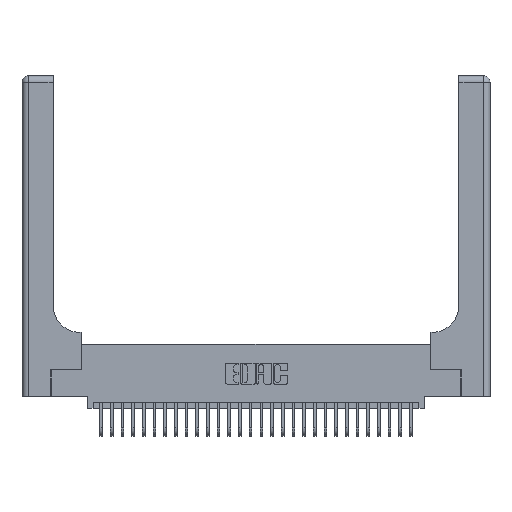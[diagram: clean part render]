
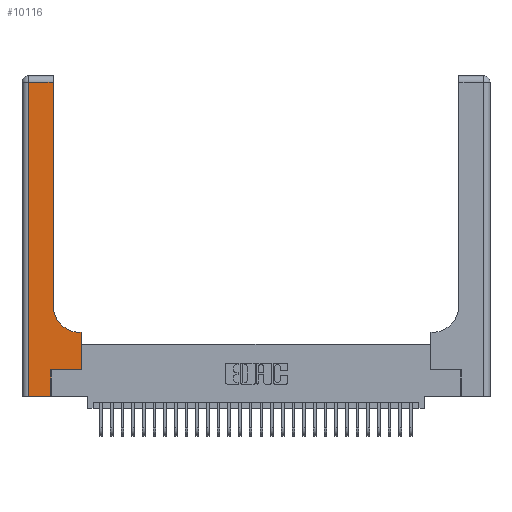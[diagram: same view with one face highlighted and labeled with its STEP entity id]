
A CAD part, top view. The second image highlights one B-rep face of the part: STEP entity #10116.
In plain terms, the highlighted planar face has unit normal (0, 0, 1).
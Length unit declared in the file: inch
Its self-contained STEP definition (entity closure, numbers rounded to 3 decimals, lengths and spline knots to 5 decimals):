
#87 = EDGE_CURVE ( 'NONE', #29212, #15285, #19806, .T. ) ;
#368 = VERTEX_POINT ( 'NONE', #7035 ) ;
#499 = EDGE_CURVE ( 'NONE', #4516, #5817, #8561, .T. ) ;
#904 = ORIENTED_EDGE ( 'NONE', *, *, #6698, .T. ) ;
#1080 = ORIENTED_EDGE ( 'NONE', *, *, #13180, .T. ) ;
#1285 = CARTESIAN_POINT ( 'NONE',  ( 0.5585, 0.6, 0.37 ) ) ;
#1563 = CARTESIAN_POINT ( 'NONE',  ( 0.5415, 0.6, 0.37 ) ) ;
#2894 = DIRECTION ( 'NONE',  ( 0., 0., -1. ) ) ;
#2907 = VERTEX_POINT ( 'NONE', #31944 ) ;
#3461 = DIRECTION ( 'NONE',  ( -1., 0., 0. ) ) ;
#3591 = CARTESIAN_POINT ( 'NONE',  ( 0.5415, 0.85, 0.37 ) ) ;
#4261 = EDGE_CURVE ( 'NONE', #13746, #29212, #31647, .T. ) ;
#4516 = VERTEX_POINT ( 'NONE', #1285 ) ;
#4831 = CARTESIAN_POINT ( 'NONE',  ( 0., 2.94, 0.37 ) ) ;
#5466 = DIRECTION ( 'NONE',  ( 0., -1., 0. ) ) ;
#5582 = VECTOR ( 'NONE', #17116, 39.37008 ) ;
#5611 = CARTESIAN_POINT ( 'NONE',  ( 0., 3., 0.37 ) ) ;
#5817 = VERTEX_POINT ( 'NONE', #1563 ) ;
#6345 = ORIENTED_EDGE ( 'NONE', *, *, #29522, .T. ) ;
#6505 = AXIS2_PLACEMENT_3D ( 'NONE', #5611, #2894, #20474 ) ;
#6698 = EDGE_CURVE ( 'NONE', #368, #2907, #15190, .T. ) ;
#6971 = CARTESIAN_POINT ( 'NONE',  ( 0.2915, 3., 0.37 ) ) ;
#7035 = CARTESIAN_POINT ( 'NONE',  ( 0.269, 0., 0.37 ) ) ;
#7038 = VERTEX_POINT ( 'NONE', #13285 ) ;
#7787 = VECTOR ( 'NONE', #3461, 39.37008 ) ;
#7920 = EDGE_LOOP ( 'NONE', ( #15923, #23489, #28900, #8496, #904, #1080, #6345, #16063, #27924 ) ) ;
#8440 = CARTESIAN_POINT ( 'NONE',  ( 0.06, 0., 0.37 ) ) ;
#8454 = DIRECTION ( 'NONE',  ( 1., 0., 0. ) ) ;
#8496 = ORIENTED_EDGE ( 'NONE', *, *, #20992, .T. ) ;
#8561 = LINE ( 'NONE', #10183, #7787 ) ;
#8568 = EDGE_CURVE ( 'NONE', #7038, #13746, #18538, .T. ) ;
#9649 = EDGE_CURVE ( 'NONE', #5817, #7038, #30574, .T. ) ;
#10116 = ADVANCED_FACE ( 'NONE', ( #22393 ), #25589, .F. ) ;
#10125 = CARTESIAN_POINT ( 'NONE',  ( 0.06, 3., 0.37 ) ) ;
#10183 = CARTESIAN_POINT ( 'NONE',  ( 0.2915, 0.6, 0.37 ) ) ;
#10711 = CARTESIAN_POINT ( 'NONE',  ( 0.269, 0.25, 0.37 ) ) ;
#10774 = VECTOR ( 'NONE', #24362, 39.37008 ) ;
#12147 = CARTESIAN_POINT ( 'NONE',  ( 0., 0., 0.37 ) ) ;
#12483 = VECTOR ( 'NONE', #8454, 39.37008 ) ;
#12898 = CARTESIAN_POINT ( 'NONE',  ( 0.06, 2.94, 0.37 ) ) ;
#13016 = VECTOR ( 'NONE', #24510, 39.37008 ) ;
#13180 = EDGE_CURVE ( 'NONE', #2907, #31056, #19071, .T. ) ;
#13285 = CARTESIAN_POINT ( 'NONE',  ( 0.2915, 0.85, 0.37 ) ) ;
#13746 = VERTEX_POINT ( 'NONE', #24627 ) ;
#15190 = LINE ( 'NONE', #26172, #16334 ) ;
#15285 = VERTEX_POINT ( 'NONE', #8440 ) ;
#15470 = VECTOR ( 'NONE', #29166, 39.37008 ) ;
#15923 = ORIENTED_EDGE ( 'NONE', *, *, #8568, .T. ) ;
#16063 = ORIENTED_EDGE ( 'NONE', *, *, #499, .T. ) ;
#16334 = VECTOR ( 'NONE', #23808, 39.37008 ) ;
#17116 = DIRECTION ( 'NONE',  ( 1., 0., 0. ) ) ;
#18538 = LINE ( 'NONE', #6971, #10774 ) ;
#19071 = LINE ( 'NONE', #10711, #12483 ) ;
#19806 = LINE ( 'NONE', #10125, #23311 ) ;
#20474 = DIRECTION ( 'NONE',  ( -1., 0., 0. ) ) ;
#20992 = EDGE_CURVE ( 'NONE', #15285, #368, #27721, .T. ) ;
#22393 = FACE_OUTER_BOUND ( 'NONE', #7920, .T. ) ;
#22466 = LINE ( 'NONE', #24207, #15470 ) ;
#23311 = VECTOR ( 'NONE', #5466, 39.37008 ) ;
#23489 = ORIENTED_EDGE ( 'NONE', *, *, #4261, .T. ) ;
#23808 = DIRECTION ( 'NONE',  ( 0., 1., 0. ) ) ;
#24207 = CARTESIAN_POINT ( 'NONE',  ( 0.5585, 0.25, 0.37 ) ) ;
#24362 = DIRECTION ( 'NONE',  ( 0., 1., 0. ) ) ;
#24510 = DIRECTION ( 'NONE',  ( -1., 0., 0. ) ) ;
#24627 = CARTESIAN_POINT ( 'NONE',  ( 0.2915, 2.94, 0.37 ) ) ;
#25499 = DIRECTION ( 'NONE',  ( 0., 0., -1. ) ) ;
#25589 = PLANE ( 'NONE',  #6505 ) ;
#26172 = CARTESIAN_POINT ( 'NONE',  ( 0.269, 0., 0.37 ) ) ;
#27113 = CARTESIAN_POINT ( 'NONE',  ( 0.5585, 0.25, 0.37 ) ) ;
#27721 = LINE ( 'NONE', #12147, #5582 ) ;
#27924 = ORIENTED_EDGE ( 'NONE', *, *, #9649, .T. ) ;
#27990 = DIRECTION ( 'NONE',  ( 1., 0., 0. ) ) ;
#28900 = ORIENTED_EDGE ( 'NONE', *, *, #87, .T. ) ;
#29166 = DIRECTION ( 'NONE',  ( 0., 1., 0. ) ) ;
#29212 = VERTEX_POINT ( 'NONE', #12898 ) ;
#29522 = EDGE_CURVE ( 'NONE', #31056, #4516, #22466, .T. ) ;
#30574 = CIRCLE ( 'NONE', #31459, 0.25 ) ;
#31056 = VERTEX_POINT ( 'NONE', #27113 ) ;
#31459 = AXIS2_PLACEMENT_3D ( 'NONE', #3591, #25499, #27990 ) ;
#31647 = LINE ( 'NONE', #4831, #13016 ) ;
#31944 = CARTESIAN_POINT ( 'NONE',  ( 0.269, 0.25, 0.37 ) ) ;
